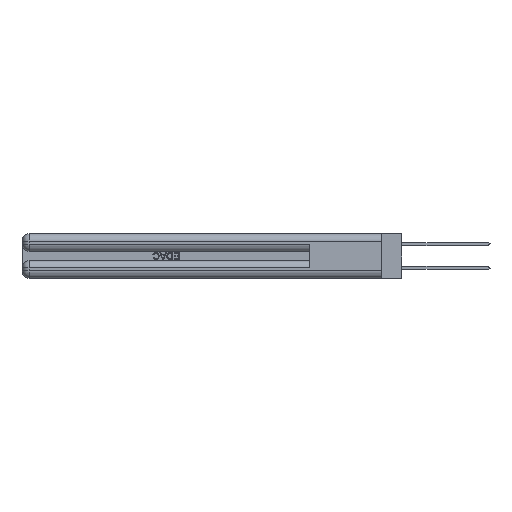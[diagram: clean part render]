
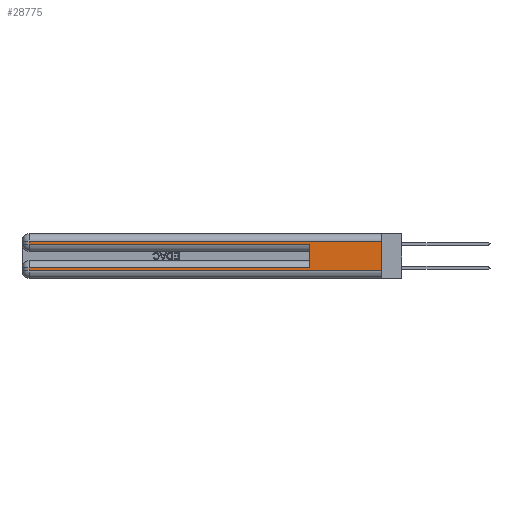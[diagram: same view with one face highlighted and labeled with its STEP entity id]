
A CAD part, left-side view. The second image highlights one B-rep face of the part: STEP entity #28775.
In plain terms, the highlighted planar face has unit normal (-1, 0, 0).
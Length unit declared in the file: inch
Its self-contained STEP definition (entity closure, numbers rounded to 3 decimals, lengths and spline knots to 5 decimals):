
#158 = CARTESIAN_POINT ( 'NONE',  ( 0., 0.6, 0.145 ) ) ;
#1928 = CARTESIAN_POINT ( 'NONE',  ( 0., 0., 0.37 ) ) ;
#1966 = LINE ( 'NONE', #37602, #23982 ) ;
#2418 = VECTOR ( 'NONE', #5837, 39.37008 ) ;
#3079 = ORIENTED_EDGE ( 'NONE', *, *, #43913, .T. ) ;
#4003 = CARTESIAN_POINT ( 'NONE',  ( 0., 0., 0.31 ) ) ;
#4097 = DIRECTION ( 'NONE',  ( 0., 0., 1. ) ) ;
#4248 = DIRECTION ( 'NONE',  ( 1., 0., 0. ) ) ;
#4859 = LINE ( 'NONE', #1928, #2418 ) ;
#5837 = DIRECTION ( 'NONE',  ( 0., 0., -1. ) ) ;
#6280 = VECTOR ( 'NONE', #36903, 39.37008 ) ;
#9436 = VERTEX_POINT ( 'NONE', #45202 ) ;
#10192 = AXIS2_PLACEMENT_3D ( 'NONE', #27598, #4248, #31450 ) ;
#10564 = DIRECTION ( 'NONE',  ( 0., -1., 0. ) ) ;
#10629 = VERTEX_POINT ( 'NONE', #22382 ) ;
#12111 = ORIENTED_EDGE ( 'NONE', *, *, #12300, .F. ) ;
#12149 = CARTESIAN_POINT ( 'NONE',  ( 0., 0.6, 0.085 ) ) ;
#12214 = VECTOR ( 'NONE', #45986, 39.37008 ) ;
#12300 = EDGE_CURVE ( 'NONE', #14739, #49197, #32135, .T. ) ;
#12925 = CARTESIAN_POINT ( 'NONE',  ( 0., 2.94, 0.06 ) ) ;
#13654 = VECTOR ( 'NONE', #16340, 39.37008 ) ;
#14100 = VERTEX_POINT ( 'NONE', #15933 ) ;
#14676 = LINE ( 'NONE', #4003, #43011 ) ;
#14739 = VERTEX_POINT ( 'NONE', #12149 ) ;
#14769 = EDGE_CURVE ( 'NONE', #14739, #10629, #23279, .T. ) ;
#15891 = PLANE ( 'NONE',  #10192 ) ;
#15933 = CARTESIAN_POINT ( 'NONE',  ( 0., 0., 0.31 ) ) ;
#15970 = DIRECTION ( 'NONE',  ( 0., 1., 0. ) ) ;
#16340 = DIRECTION ( 'NONE',  ( 0., 0., -1. ) ) ;
#16558 = ORIENTED_EDGE ( 'NONE', *, *, #20559, .T. ) ;
#18505 = VERTEX_POINT ( 'NONE', #42117 ) ;
#19183 = CARTESIAN_POINT ( 'NONE',  ( 0., 2.94, 0.37 ) ) ;
#19490 = VECTOR ( 'NONE', #4097, 39.37008 ) ;
#20182 = DIRECTION ( 'NONE',  ( 0., 1., 0. ) ) ;
#20275 = CARTESIAN_POINT ( 'NONE',  ( 0., 2.94, 0.37 ) ) ;
#20374 = ORIENTED_EDGE ( 'NONE', *, *, #14769, .T. ) ;
#20559 = EDGE_CURVE ( 'NONE', #33655, #18505, #1966, .T. ) ;
#21473 = CARTESIAN_POINT ( 'NONE',  ( 0., 0., 0.285 ) ) ;
#21978 = CARTESIAN_POINT ( 'NONE',  ( 0., 2.94, 0.31 ) ) ;
#22329 = FACE_OUTER_BOUND ( 'NONE', #44452, .T. ) ;
#22382 = CARTESIAN_POINT ( 'NONE',  ( 0., 2.94, 0.085 ) ) ;
#23004 = EDGE_CURVE ( 'NONE', #9436, #49197, #37199, .T. ) ;
#23279 = LINE ( 'NONE', #46968, #25687 ) ;
#23982 = VECTOR ( 'NONE', #10564, 39.37008 ) ;
#25332 = EDGE_CURVE ( 'NONE', #14100, #47587, #14676, .T. ) ;
#25554 = EDGE_CURVE ( 'NONE', #14100, #18505, #4859, .T. ) ;
#25687 = VECTOR ( 'NONE', #20182, 39.37008 ) ;
#25787 = EDGE_CURVE ( 'NONE', #47587, #9436, #32786, .T. ) ;
#27021 = ORIENTED_EDGE ( 'NONE', *, *, #25332, .T. ) ;
#27598 = CARTESIAN_POINT ( 'NONE',  ( 0., 0., 0.37 ) ) ;
#28775 = ADVANCED_FACE ( 'NONE', ( #22329 ), #15891, .F. ) ;
#31450 = DIRECTION ( 'NONE',  ( 0., 0., -1. ) ) ;
#32135 = LINE ( 'NONE', #158, #19490 ) ;
#32786 = LINE ( 'NONE', #19183, #12214 ) ;
#33655 = VERTEX_POINT ( 'NONE', #12925 ) ;
#36903 = DIRECTION ( 'NONE',  ( 0., -1., 0. ) ) ;
#37199 = LINE ( 'NONE', #21473, #6280 ) ;
#37602 = CARTESIAN_POINT ( 'NONE',  ( 0., 0., 0.06 ) ) ;
#39064 = CARTESIAN_POINT ( 'NONE',  ( 0., 0.6, 0.285 ) ) ;
#42117 = CARTESIAN_POINT ( 'NONE',  ( 0., 0., 0.06 ) ) ;
#43011 = VECTOR ( 'NONE', #15970, 39.37008 ) ;
#43913 = EDGE_CURVE ( 'NONE', #10629, #33655, #44363, .T. ) ;
#43926 = ORIENTED_EDGE ( 'NONE', *, *, #25554, .F. ) ;
#44363 = LINE ( 'NONE', #20275, #13654 ) ;
#44452 = EDGE_LOOP ( 'NONE', ( #43926, #27021, #47692, #46606, #12111, #20374, #3079, #16558 ) ) ;
#45202 = CARTESIAN_POINT ( 'NONE',  ( 0., 2.94, 0.285 ) ) ;
#45986 = DIRECTION ( 'NONE',  ( 0., 0., -1. ) ) ;
#46606 = ORIENTED_EDGE ( 'NONE', *, *, #23004, .T. ) ;
#46968 = CARTESIAN_POINT ( 'NONE',  ( 0., 0., 0.085 ) ) ;
#47587 = VERTEX_POINT ( 'NONE', #21978 ) ;
#47692 = ORIENTED_EDGE ( 'NONE', *, *, #25787, .T. ) ;
#49197 = VERTEX_POINT ( 'NONE', #39064 ) ;
